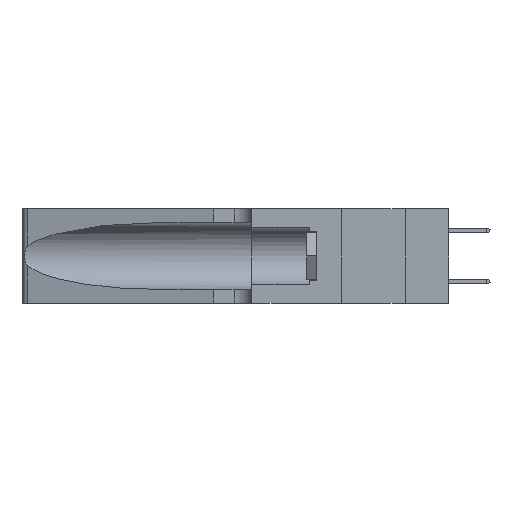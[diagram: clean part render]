
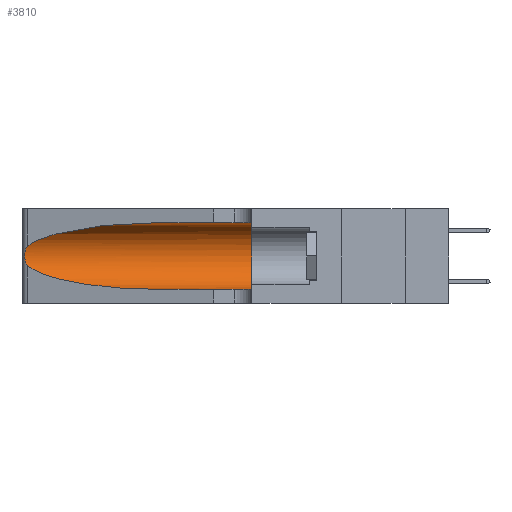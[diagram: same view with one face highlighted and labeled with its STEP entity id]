
A CAD part, left-side view. The second image highlights one B-rep face of the part: STEP entity #3810.
In plain terms, the highlighted cylindrical face has radius 3.308 mm (diameter 6.617 mm), a partial arc.
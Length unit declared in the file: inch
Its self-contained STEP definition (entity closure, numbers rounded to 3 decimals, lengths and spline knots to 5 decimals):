
#528 = CARTESIAN_POINT ( 'NONE',  ( 0.25555, 1.22994, 0.2215 ) ) ;
#597 = CARTESIAN_POINT ( 'NONE',  ( 0.25789, 1.23486, 0.15765 ) ) ;
#1194 = ORIENTED_EDGE ( 'NONE', *, *, #4432, .T. ) ;
#1481 = CARTESIAN_POINT ( 'NONE',  ( 0.1305, 0.35, 0.185 ) ) ;
#1997 = CYLINDRICAL_SURFACE ( 'NONE', #13559, 0.13025 ) ;
#2165 = CARTESIAN_POINT ( 'NONE',  ( 0.25555, 1.22993, 0.14849 ) ) ;
#2269 = CARTESIAN_POINT ( 'NONE',  ( 0.1305, 0.72297, 0.31525 ) ) ;
#2293 = VERTEX_POINT ( 'NONE', #11158 ) ;
#2357 = CARTESIAN_POINT ( 'NONE',  ( 0.18966, 0.96281, 0.31525 ) ) ;
#2453 = DIRECTION ( 'NONE',  ( 0., 0., -1. ) ) ;
#2524 = DIRECTION ( 'NONE',  ( 0., -1., 0. ) ) ;
#2821 = AXIS2_PLACEMENT_3D ( 'NONE', #1481, #12337, #3045 ) ;
#3045 = DIRECTION ( 'NONE',  ( 0., 0., 1. ) ) ;
#3343 = CARTESIAN_POINT ( 'NONE',  ( 0.1305, 1.61858, 0.31525 ) ) ;
#3441 = CARTESIAN_POINT ( 'NONE',  ( 0.2373, 1.15595, 0.08982 ) ) ;
#3492 = EDGE_CURVE ( 'NONE', #6717, #4237, #8465, .T. ) ;
#3703 = CIRCLE ( 'NONE', #2821, 0.13025 ) ;
#3810 = ADVANCED_FACE ( 'NONE', ( #14290 ), #1997, .F. ) ;
#3861 = VERTEX_POINT ( 'NONE', #16378 ) ;
#4028 = EDGE_CURVE ( 'NONE', #4237, #4806, #3703, .T. ) ;
#4152 = DIRECTION ( 'NONE',  ( 0., -1., 0. ) ) ;
#4235 = VECTOR ( 'NONE', #15597, 39.37008 ) ;
#4237 = VERTEX_POINT ( 'NONE', #14278 ) ;
#4432 = EDGE_CURVE ( 'NONE', #6717, #11634, #5226, .T. ) ;
#4806 = VERTEX_POINT ( 'NONE', #15475 ) ;
#5059 = CARTESIAN_POINT ( 'NONE',  ( 0.1305, 0.72297, 0.05475 ) ) ;
#5226 =( BOUNDED_CURVE ( )  B_SPLINE_CURVE ( 3, ( #5572, #2357, #10178, #16161 ),
 .UNSPECIFIED., .F., .F. ) 
 B_SPLINE_CURVE_WITH_KNOTS ( ( 4, 4 ),
 ( 1.5708, 2.84003 ),
 .UNSPECIFIED. ) 
 CURVE ( )  GEOMETRIC_REPRESENTATION_ITEM ( )  RATIONAL_B_SPLINE_CURVE ( ( 1., 0.87, 0.87, 1. ) ) 
 REPRESENTATION_ITEM ( '' )  );
#5306 = CARTESIAN_POINT ( 'NONE',  ( 0.25787, 1.23484, 0.2124 ) ) ;
#5572 = CARTESIAN_POINT ( 'NONE',  ( 0.1305, 0.72297, 0.31525 ) ) ;
#6178 = EDGE_CURVE ( 'NONE', #2293, #4806, #18012, .T. ) ;
#6364 =( BOUNDED_CURVE ( )  B_SPLINE_CURVE ( 3, ( #11218, #3441, #14198, #5059 ),
 .UNSPECIFIED., .F., .F. ) 
 B_SPLINE_CURVE_WITH_KNOTS ( ( 4, 4 ),
 ( 3.44316, 4.71239 ),
 .UNSPECIFIED. ) 
 CURVE ( )  GEOMETRIC_REPRESENTATION_ITEM ( )  RATIONAL_B_SPLINE_CURVE ( ( 1., 0.87, 0.87, 1. ) ) 
 REPRESENTATION_ITEM ( '' )  );
#6717 = VERTEX_POINT ( 'NONE', #2269 ) ;
#6891 = CARTESIAN_POINT ( 'NONE',  ( 0.26018, 1.23835, 0.19895 ) ) ;
#8465 = LINE ( 'NONE', #3343, #4235 ) ;
#8481 = CARTESIAN_POINT ( 'NONE',  ( 0.26075, 1.23896, 0.178 ) ) ;
#8990 = ORIENTED_EDGE ( 'NONE', *, *, #19522, .T. ) ;
#9040 = ORIENTED_EDGE ( 'NONE', *, *, #3492, .F. ) ;
#9990 = CARTESIAN_POINT ( 'NONE',  ( 0.25856, 1.23593, 0.16098 ) ) ;
#10178 = CARTESIAN_POINT ( 'NONE',  ( 0.2373, 1.15595, 0.28018 ) ) ;
#10553 = ORIENTED_EDGE ( 'NONE', *, *, #6178, .T. ) ;
#11158 = CARTESIAN_POINT ( 'NONE',  ( 0.1305, 0.72297, 0.05475 ) ) ;
#11218 = CARTESIAN_POINT ( 'NONE',  ( 0.25487, 1.22718, 0.14631 ) ) ;
#11503 = CARTESIAN_POINT ( 'NONE',  ( 0.25639, 1.23186, 0.15144 ) ) ;
#11617 = EDGE_CURVE ( 'NONE', #11634, #3861, #19700, .T. ) ;
#11634 = VERTEX_POINT ( 'NONE', #14482 ) ;
#11774 = ORIENTED_EDGE ( 'NONE', *, *, #11617, .T. ) ;
#11837 = CARTESIAN_POINT ( 'NONE',  ( 0.1305, 1.61858, 0.185 ) ) ;
#12337 = DIRECTION ( 'NONE',  ( 0., 1., 0. ) ) ;
#12925 = CARTESIAN_POINT ( 'NONE',  ( 0.25487, 1.22718, 0.22369 ) ) ;
#12986 = CARTESIAN_POINT ( 'NONE',  ( 0.25487, 1.22718, 0.14631 ) ) ;
#13378 = CARTESIAN_POINT ( 'NONE',  ( 0.1305, 1.61858, 0.05475 ) ) ;
#13559 = AXIS2_PLACEMENT_3D ( 'NONE', #11837, #2524, #2453 ) ;
#13603 = VECTOR ( 'NONE', #4152, 39.37008 ) ;
#14198 = CARTESIAN_POINT ( 'NONE',  ( 0.18966, 0.96281, 0.05475 ) ) ;
#14278 = CARTESIAN_POINT ( 'NONE',  ( 0.1305, 0.35, 0.31525 ) ) ;
#14290 = FACE_OUTER_BOUND ( 'NONE', #16453, .T. ) ;
#14420 = CARTESIAN_POINT ( 'NONE',  ( 0.25639, 1.23184, 0.21858 ) ) ;
#14482 = CARTESIAN_POINT ( 'NONE',  ( 0.25487, 1.22718, 0.22369 ) ) ;
#15475 = CARTESIAN_POINT ( 'NONE',  ( 0.1305, 0.35, 0.05475 ) ) ;
#15597 = DIRECTION ( 'NONE',  ( 0., -1., 0. ) ) ;
#15900 = CARTESIAN_POINT ( 'NONE',  ( 0.25854, 1.2359, 0.20912 ) ) ;
#16161 = CARTESIAN_POINT ( 'NONE',  ( 0.25487, 1.22718, 0.22369 ) ) ;
#16378 = CARTESIAN_POINT ( 'NONE',  ( 0.25487, 1.22718, 0.14631 ) ) ;
#16453 = EDGE_LOOP ( 'NONE', ( #1194, #11774, #8990, #10553, #18563, #9040 ) ) ;
#17383 = CARTESIAN_POINT ( 'NONE',  ( 0.26075, 1.23896, 0.19203 ) ) ;
#18012 = LINE ( 'NONE', #13378, #13603 ) ;
#18563 = ORIENTED_EDGE ( 'NONE', *, *, #4028, .F. ) ;
#18897 = CARTESIAN_POINT ( 'NONE',  ( 0.26017, 1.23833, 0.17102 ) ) ;
#19522 = EDGE_CURVE ( 'NONE', #3861, #2293, #6364, .T. ) ;
#19700 = B_SPLINE_CURVE_WITH_KNOTS ( 'NONE', 3,
 ( #12925, #528, #14420, #5306, #15900, #6891, #17383, #8481, #18897, #9990, #597, #11503, #2165, #12986 ),
 .UNSPECIFIED., .F., .F.,
 ( 4, 2, 2, 2, 2, 2, 4 ),
 ( 0., 0.00027, 0.00053, 0.00107, 0.0016, 0.00187, 0.00214 ),
 .UNSPECIFIED. ) ;
